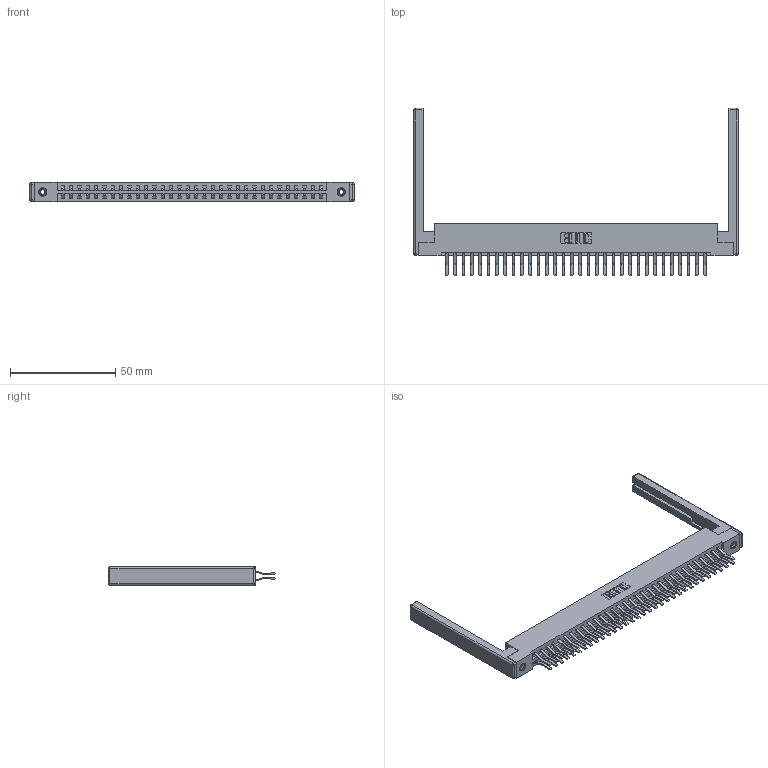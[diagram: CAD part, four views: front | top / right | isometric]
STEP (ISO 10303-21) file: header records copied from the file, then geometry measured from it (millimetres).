
FILE_DESCRIPTION (( 'STEP AP203' ), '1' );
FILE_NAME ('337-064-560-268.STEP', '2019-10-09T22:46:25', ( '' ), ( '' ), 'SwSTEP 2.0', 'SolidWorks 2016', '' );
FILE_SCHEMA (( 'CONFIG_CONTROL_DESIGN' ));
Length unit declared in the file: inch
Products named in the file (5): 337-064-560-268; 345-250-001_345-250-001-102; 337 Part_Flush Mounting Lugs - 0.156 Dia-TI; 345-292-001_560 Tail; 307-220-068
Assembly tree (69 placements, depth 2):
  337-064-560-268
    337 Part_Flush Mounting Lugs - 0.156 Dia-TI
    345-292-001_560 Tail  x64
    345-250-001_345-250-001-102  x2
    307-220-068  x2
Bounding box: 154.23 x 79.52 x 9.4 mm (x, y, z)
Volume: 20925 mm3; surface area: 23850.1 mm2
Topology: 69 solids, 69 shells, 3852 faces, 11389 edges, 7486 vertices
Faces by surface type: plane 2590, cylinder 1238, cone 12, sphere 8, torus 4
Entity records: 28952 total; most frequent: CARTESIAN_POINT 4851, ORIENTED_EDGE 4776, DIRECTION 4218, EDGE_CURVE 2388, LINE 2206, VECTOR 2206, VERTEX_POINT 1582, AXIS2_PLACEMENT_3D 1006
